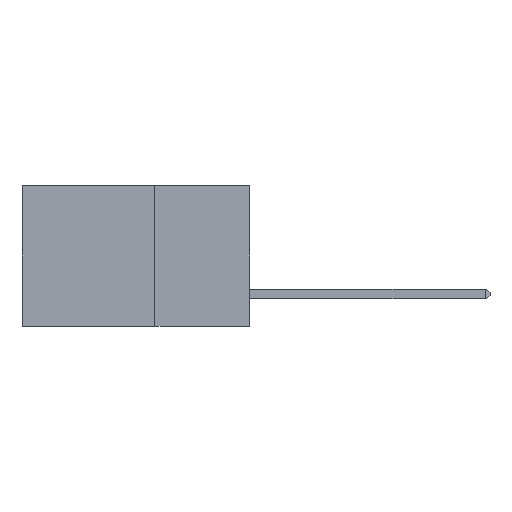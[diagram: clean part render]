
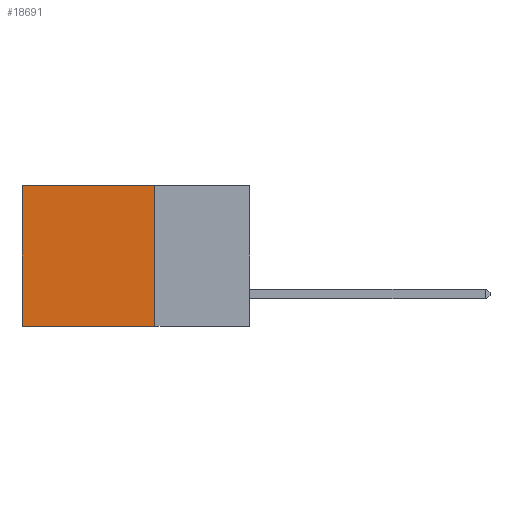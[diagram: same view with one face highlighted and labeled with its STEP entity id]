
A CAD part, left-side view. The second image highlights one B-rep face of the part: STEP entity #18691.
In plain terms, the highlighted planar face has unit normal (-1, 0, 0).
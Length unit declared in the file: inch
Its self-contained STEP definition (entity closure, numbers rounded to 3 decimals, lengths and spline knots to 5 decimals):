
#713 = AXIS2_PLACEMENT_3D ( 'NONE', #8463, #20138, #10139 ) ;
#1217 = ORIENTED_EDGE ( 'NONE', *, *, #15764, .T. ) ;
#1801 = VECTOR ( 'NONE', #7923, 39.37008 ) ;
#2363 = CARTESIAN_POINT ( 'NONE',  ( 0.2875, 0.6, -0.37 ) ) ;
#2543 = CARTESIAN_POINT ( 'NONE',  ( 0.2875, 0.25, -0.37 ) ) ;
#2621 = VERTEX_POINT ( 'NONE', #2363 ) ;
#2910 = CARTESIAN_POINT ( 'NONE',  ( 0.2875, 0.25, 0. ) ) ;
#3195 = ORIENTED_EDGE ( 'NONE', *, *, #11022, .F. ) ;
#3707 = LINE ( 'NONE', #5423, #12670 ) ;
#3947 = VECTOR ( 'NONE', #7964, 39.37008 ) ;
#4378 = ORIENTED_EDGE ( 'NONE', *, *, #8311, .T. ) ;
#4731 = FACE_OUTER_BOUND ( 'NONE', #17868, .T. ) ;
#5423 = CARTESIAN_POINT ( 'NONE',  ( 0.2875, 0.25, 0. ) ) ;
#7923 = DIRECTION ( 'NONE',  ( 0., 1., 0. ) ) ;
#7964 = DIRECTION ( 'NONE',  ( 0., 0., -1. ) ) ;
#8311 = EDGE_CURVE ( 'NONE', #14744, #2621, #21270, .T. ) ;
#8463 = CARTESIAN_POINT ( 'NONE',  ( 0.2875, 0.25, 0. ) ) ;
#8794 = DIRECTION ( 'NONE',  ( 0., 1., 0. ) ) ;
#8969 = LINE ( 'NONE', #2910, #3947 ) ;
#9247 = EDGE_CURVE ( 'NONE', #10886, #2621, #15727, .T. ) ;
#10139 = DIRECTION ( 'NONE',  ( 0., 0., -1. ) ) ;
#10886 = VERTEX_POINT ( 'NONE', #2543 ) ;
#11022 = EDGE_CURVE ( 'NONE', #13829, #10886, #8969, .T. ) ;
#11857 = CARTESIAN_POINT ( 'NONE',  ( 0.2875, 0.25, 0. ) ) ;
#12670 = VECTOR ( 'NONE', #8794, 39.37008 ) ;
#13829 = VERTEX_POINT ( 'NONE', #11857 ) ;
#14744 = VERTEX_POINT ( 'NONE', #17499 ) ;
#15727 = LINE ( 'NONE', #17892, #1801 ) ;
#15764 = EDGE_CURVE ( 'NONE', #13829, #14744, #3707, .T. ) ;
#16812 = VECTOR ( 'NONE', #20494, 39.37008 ) ;
#17499 = CARTESIAN_POINT ( 'NONE',  ( 0.2875, 0.6, 0. ) ) ;
#17868 = EDGE_LOOP ( 'NONE', ( #4378, #21172, #3195, #1217 ) ) ;
#17892 = CARTESIAN_POINT ( 'NONE',  ( 0.2875, 0.25, -0.37 ) ) ;
#18691 = ADVANCED_FACE ( 'NONE', ( #4731 ), #21730, .F. ) ;
#18794 = CARTESIAN_POINT ( 'NONE',  ( 0.2875, 0.6, 0. ) ) ;
#20138 = DIRECTION ( 'NONE',  ( 1., 0., 0. ) ) ;
#20494 = DIRECTION ( 'NONE',  ( 0., 0., -1. ) ) ;
#21172 = ORIENTED_EDGE ( 'NONE', *, *, #9247, .F. ) ;
#21270 = LINE ( 'NONE', #18794, #16812 ) ;
#21730 = PLANE ( 'NONE',  #713 ) ;
